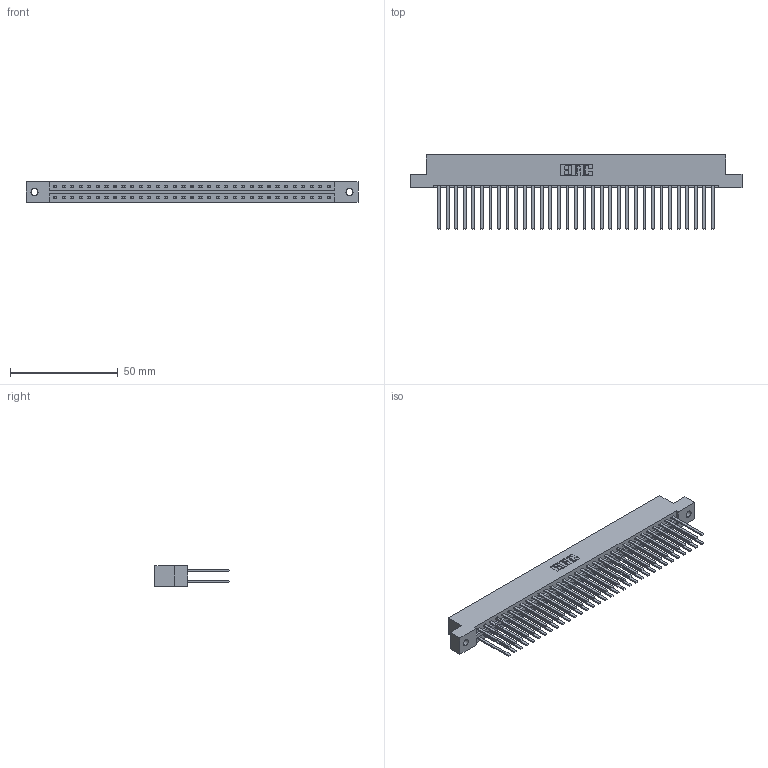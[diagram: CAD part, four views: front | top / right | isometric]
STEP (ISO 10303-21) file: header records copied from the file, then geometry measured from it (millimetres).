
FILE_DESCRIPTION (( 'STEP AP203' ), '1' );
FILE_NAME ('387-066-544-202.STEP', '2018-09-21T10:20:10', ( '' ), ( '' ), 'SwSTEP 2.0', 'SolidWorks 2016', '' );
FILE_SCHEMA (( 'CONFIG_CONTROL_DESIGN' ));
Length unit declared in the file: inch
Products named in the file (3): 337 Part_Flush Mounting Lugs - 0.128 Dia; 345-292-001_345-293-144; 387-066-544-202
Assembly tree (67 placements, depth 2):
  387-066-544-202
    337 Part_Flush Mounting Lugs - 0.128 Dia
    345-292-001_345-293-144  x66
Bounding box: 153.77 x 34.3 x 9.4 mm (x, y, z)
Volume: 16974.4 mm3; surface area: 21851.8 mm2
Topology: 67 solids, 67 shells, 3282 faces, 9749 edges, 6410 vertices
Faces by surface type: plane 2314, cylinder 968
Entity records: 26569 total; most frequent: CARTESIAN_POINT 4482, ORIENTED_EDGE 4418, DIRECTION 3825, EDGE_CURVE 2209, LINE 2085, VECTOR 2085, VERTEX_POINT 1470, AXIS2_PLACEMENT_3D 870
